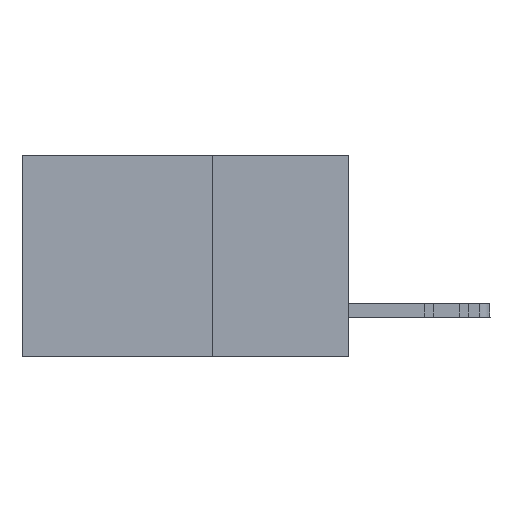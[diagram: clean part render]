
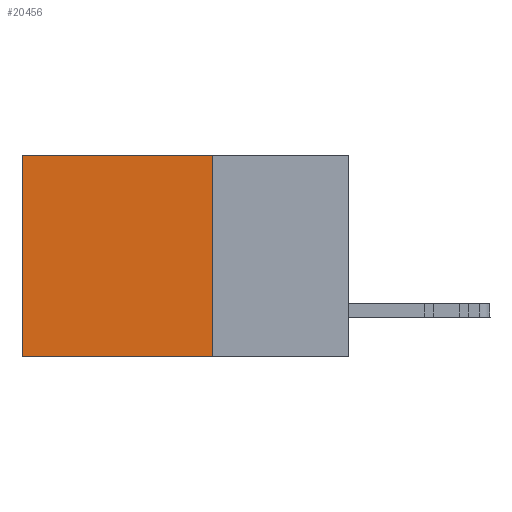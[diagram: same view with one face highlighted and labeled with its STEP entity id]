
A CAD part, left-side view. The second image highlights one B-rep face of the part: STEP entity #20456.
In plain terms, the highlighted planar face has unit normal (-1, 0, 0).
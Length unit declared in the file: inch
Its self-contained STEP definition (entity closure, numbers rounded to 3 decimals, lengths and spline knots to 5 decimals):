
#1519 = VECTOR ( 'NONE', #4768, 39.37008 ) ;
#2260 = AXIS2_PLACEMENT_3D ( 'NONE', #28303, #7095, #11734 ) ;
#4000 = VERTEX_POINT ( 'NONE', #9831 ) ;
#4768 = DIRECTION ( 'NONE',  ( 0., 1., 0. ) ) ;
#5917 = CARTESIAN_POINT ( 'NONE',  ( 0.298, 0.25, -0.37 ) ) ;
#6221 = DIRECTION ( 'NONE',  ( 0., 0., -1. ) ) ;
#7095 = DIRECTION ( 'NONE',  ( 1., 0., 0. ) ) ;
#7120 = VECTOR ( 'NONE', #6221, 39.37008 ) ;
#8619 = EDGE_LOOP ( 'NONE', ( #22826, #19261, #24553, #19499 ) ) ;
#8936 = CARTESIAN_POINT ( 'NONE',  ( 0.298, 0.25, 0. ) ) ;
#9567 = CARTESIAN_POINT ( 'NONE',  ( 0.298, 0.25, -0.37 ) ) ;
#9831 = CARTESIAN_POINT ( 'NONE',  ( 0.298, 0.6, 0. ) ) ;
#9968 = CARTESIAN_POINT ( 'NONE',  ( 0.298, 0.6, 0. ) ) ;
#11402 = VECTOR ( 'NONE', #11978, 39.37008 ) ;
#11734 = DIRECTION ( 'NONE',  ( 0., 0., -1. ) ) ;
#11747 = VERTEX_POINT ( 'NONE', #5917 ) ;
#11978 = DIRECTION ( 'NONE',  ( 0., 0., -1. ) ) ;
#13472 = CARTESIAN_POINT ( 'NONE',  ( 0.298, 0.25, 0. ) ) ;
#18159 = EDGE_CURVE ( 'NONE', #26945, #4000, #20409, .T. ) ;
#18845 = FACE_OUTER_BOUND ( 'NONE', #8619, .T. ) ;
#18936 = VECTOR ( 'NONE', #22544, 39.37008 ) ;
#18990 = EDGE_CURVE ( 'NONE', #26945, #11747, #27416, .T. ) ;
#19261 = ORIENTED_EDGE ( 'NONE', *, *, #24754, .F. ) ;
#19499 = ORIENTED_EDGE ( 'NONE', *, *, #18159, .T. ) ;
#20231 = VERTEX_POINT ( 'NONE', #26788 ) ;
#20409 = LINE ( 'NONE', #8936, #18936 ) ;
#20456 = ADVANCED_FACE ( 'NONE', ( #18845 ), #30461, .F. ) ;
#22544 = DIRECTION ( 'NONE',  ( 0., 1., 0. ) ) ;
#22826 = ORIENTED_EDGE ( 'NONE', *, *, #29952, .T. ) ;
#24439 = CARTESIAN_POINT ( 'NONE',  ( 0.298, 0.25, 0. ) ) ;
#24553 = ORIENTED_EDGE ( 'NONE', *, *, #18990, .F. ) ;
#24754 = EDGE_CURVE ( 'NONE', #11747, #20231, #25969, .T. ) ;
#25969 = LINE ( 'NONE', #9567, #1519 ) ;
#26212 = LINE ( 'NONE', #9968, #11402 ) ;
#26788 = CARTESIAN_POINT ( 'NONE',  ( 0.298, 0.6, -0.37 ) ) ;
#26945 = VERTEX_POINT ( 'NONE', #24439 ) ;
#27416 = LINE ( 'NONE', #13472, #7120 ) ;
#28303 = CARTESIAN_POINT ( 'NONE',  ( 0.298, 0.25, 0. ) ) ;
#29952 = EDGE_CURVE ( 'NONE', #4000, #20231, #26212, .T. ) ;
#30461 = PLANE ( 'NONE',  #2260 ) ;
